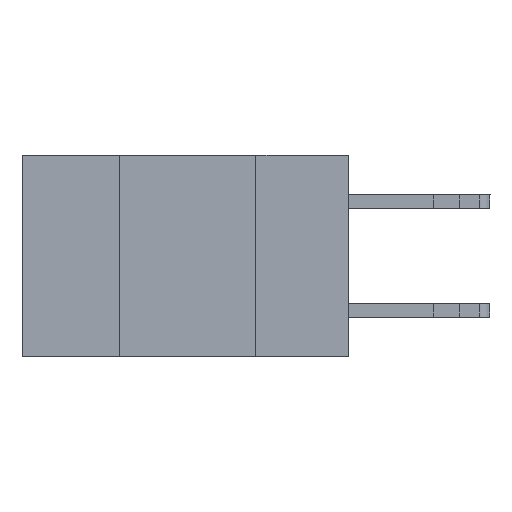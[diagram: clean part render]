
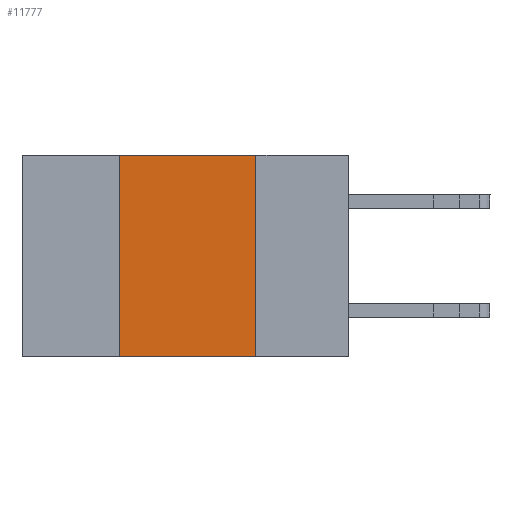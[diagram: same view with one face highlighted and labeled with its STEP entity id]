
A CAD part, left-side view. The second image highlights one B-rep face of the part: STEP entity #11777.
In plain terms, the highlighted planar face has unit normal (-1, 0, 0).
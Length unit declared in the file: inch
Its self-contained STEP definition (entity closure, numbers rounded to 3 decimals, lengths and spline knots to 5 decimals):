
#476 = VERTEX_POINT ( 'NONE', #8429 ) ;
#651 = CARTESIAN_POINT ( 'NONE',  ( 0., 0.6, 0. ) ) ;
#2434 = CARTESIAN_POINT ( 'NONE',  ( 0., 0.17, -0.37 ) ) ;
#3210 = CARTESIAN_POINT ( 'NONE',  ( 0., 0.6, 0. ) ) ;
#4459 = EDGE_CURVE ( 'NONE', #476, #18369, #12732, .T. ) ;
#4654 = DIRECTION ( 'NONE',  ( 0., 0., 1. ) ) ;
#4768 = LINE ( 'NONE', #11258, #16027 ) ;
#5849 = DIRECTION ( 'NONE',  ( 1., 0., 0. ) ) ;
#6890 = LINE ( 'NONE', #11571, #11800 ) ;
#7930 = EDGE_CURVE ( 'NONE', #18369, #12191, #8083, .T. ) ;
#8083 = LINE ( 'NONE', #3210, #9514 ) ;
#8122 = EDGE_LOOP ( 'NONE', ( #15100, #16649, #18327, #17930 ) ) ;
#8169 = DIRECTION ( 'NONE',  ( 0., 0., -1. ) ) ;
#8189 = DIRECTION ( 'NONE',  ( 0., -1., 0. ) ) ;
#8429 = CARTESIAN_POINT ( 'NONE',  ( 0., 0.42, -0.37 ) ) ;
#9514 = VECTOR ( 'NONE', #8189, 39.37008 ) ;
#10462 = AXIS2_PLACEMENT_3D ( 'NONE', #651, #5849, #12328 ) ;
#11258 = CARTESIAN_POINT ( 'NONE',  ( 0., 0.6, -0.37 ) ) ;
#11571 = CARTESIAN_POINT ( 'NONE',  ( 0., 0.17, 0. ) ) ;
#11777 = ADVANCED_FACE ( 'NONE', ( #15659 ), #18648, .F. ) ;
#11800 = VECTOR ( 'NONE', #8169, 39.37008 ) ;
#12191 = VERTEX_POINT ( 'NONE', #16798 ) ;
#12328 = DIRECTION ( 'NONE',  ( 0., 0., -1. ) ) ;
#12347 = EDGE_CURVE ( 'NONE', #476, #13458, #4768, .T. ) ;
#12732 = LINE ( 'NONE', #19236, #17030 ) ;
#13458 = VERTEX_POINT ( 'NONE', #2434 ) ;
#13746 = EDGE_CURVE ( 'NONE', #12191, #13458, #6890, .T. ) ;
#15100 = ORIENTED_EDGE ( 'NONE', *, *, #13746, .F. ) ;
#15659 = FACE_OUTER_BOUND ( 'NONE', #8122, .T. ) ;
#15829 = CARTESIAN_POINT ( 'NONE',  ( 0., 0.42, 0. ) ) ;
#15947 = DIRECTION ( 'NONE',  ( 0., -1., 0. ) ) ;
#16027 = VECTOR ( 'NONE', #15947, 39.37008 ) ;
#16649 = ORIENTED_EDGE ( 'NONE', *, *, #7930, .F. ) ;
#16798 = CARTESIAN_POINT ( 'NONE',  ( 0., 0.17, 0. ) ) ;
#17030 = VECTOR ( 'NONE', #4654, 39.37008 ) ;
#17930 = ORIENTED_EDGE ( 'NONE', *, *, #12347, .T. ) ;
#18327 = ORIENTED_EDGE ( 'NONE', *, *, #4459, .F. ) ;
#18369 = VERTEX_POINT ( 'NONE', #15829 ) ;
#18648 = PLANE ( 'NONE',  #10462 ) ;
#19236 = CARTESIAN_POINT ( 'NONE',  ( 0., 0.42, 0. ) ) ;
